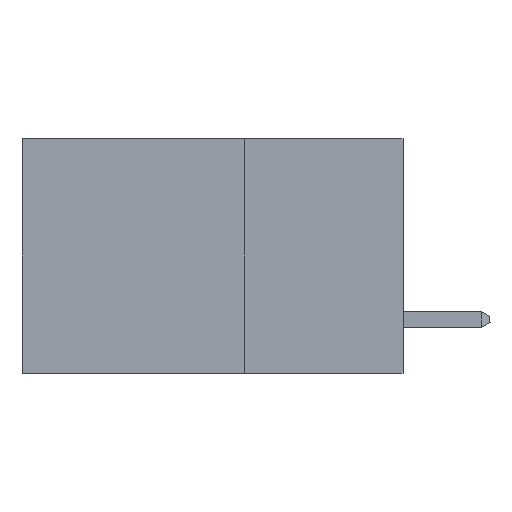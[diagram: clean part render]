
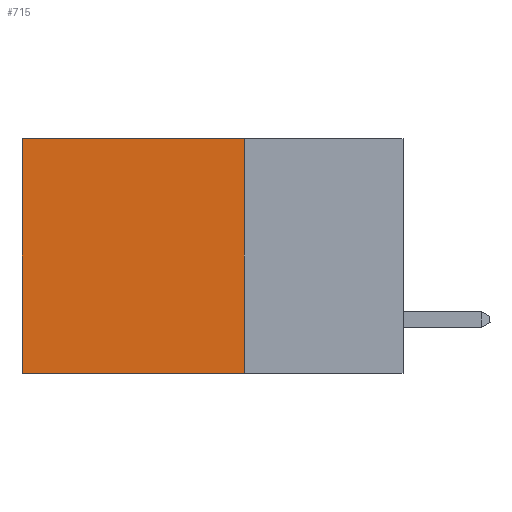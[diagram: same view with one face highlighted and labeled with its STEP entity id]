
A CAD part, left-side view. The second image highlights one B-rep face of the part: STEP entity #715.
In plain terms, the highlighted planar face has unit normal (-1, 0, 0).
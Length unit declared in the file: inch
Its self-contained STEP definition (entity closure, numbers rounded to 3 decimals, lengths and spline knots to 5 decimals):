
#684 = AXIS2_PLACEMENT_3D ( 'NONE', #42474, #21141, #42786 ) ;
#715 = ADVANCED_FACE ( 'NONE', ( #16308 ), #6292, .F. ) ;
#1144 = ORIENTED_EDGE ( 'NONE', *, *, #30104, .F. ) ;
#2700 = ORIENTED_EDGE ( 'NONE', *, *, #9098, .T. ) ;
#3795 = CARTESIAN_POINT ( 'NONE',  ( 0.2875, 0.25, 0. ) ) ;
#5429 = EDGE_CURVE ( 'NONE', #36516, #42840, #5952, .T. ) ;
#5790 = VERTEX_POINT ( 'NONE', #8399 ) ;
#5952 = LINE ( 'NONE', #10090, #33958 ) ;
#6292 = PLANE ( 'NONE',  #684 ) ;
#6444 = VECTOR ( 'NONE', #27448, 39.37008 ) ;
#6794 = CARTESIAN_POINT ( 'NONE',  ( 0.2875, 0.25, -0.37 ) ) ;
#8382 = CARTESIAN_POINT ( 'NONE',  ( 0.2875, 0.25, 0. ) ) ;
#8399 = CARTESIAN_POINT ( 'NONE',  ( 0.2875, 0.6, 0. ) ) ;
#9098 = EDGE_CURVE ( 'NONE', #36516, #5790, #30743, .T. ) ;
#10090 = CARTESIAN_POINT ( 'NONE',  ( 0.2875, 0.25, 0. ) ) ;
#16308 = FACE_OUTER_BOUND ( 'NONE', #29514, .T. ) ;
#16380 = CARTESIAN_POINT ( 'NONE',  ( 0.2875, 0.25, -0.37 ) ) ;
#17772 = ORIENTED_EDGE ( 'NONE', *, *, #23701, .T. ) ;
#19584 = CARTESIAN_POINT ( 'NONE',  ( 0.2875, 0.6, -0.37 ) ) ;
#21088 = CARTESIAN_POINT ( 'NONE',  ( 0.2875, 0.6, 0. ) ) ;
#21141 = DIRECTION ( 'NONE',  ( 1., 0., 0. ) ) ;
#21307 = VECTOR ( 'NONE', #22705, 39.37008 ) ;
#22705 = DIRECTION ( 'NONE',  ( 0., 1., 0. ) ) ;
#23375 = VERTEX_POINT ( 'NONE', #19584 ) ;
#23701 = EDGE_CURVE ( 'NONE', #5790, #23375, #35335, .T. ) ;
#27265 = DIRECTION ( 'NONE',  ( 0., 0., -1. ) ) ;
#27448 = DIRECTION ( 'NONE',  ( 0., 1., 0. ) ) ;
#28125 = DIRECTION ( 'NONE',  ( 0., 0., -1. ) ) ;
#29514 = EDGE_LOOP ( 'NONE', ( #17772, #1144, #42038, #2700 ) ) ;
#30104 = EDGE_CURVE ( 'NONE', #42840, #23375, #44038, .T. ) ;
#30743 = LINE ( 'NONE', #8382, #21307 ) ;
#33958 = VECTOR ( 'NONE', #27265, 39.37008 ) ;
#35335 = LINE ( 'NONE', #21088, #39256 ) ;
#36516 = VERTEX_POINT ( 'NONE', #3795 ) ;
#39256 = VECTOR ( 'NONE', #28125, 39.37008 ) ;
#42038 = ORIENTED_EDGE ( 'NONE', *, *, #5429, .F. ) ;
#42474 = CARTESIAN_POINT ( 'NONE',  ( 0.2875, 0.25, 0. ) ) ;
#42786 = DIRECTION ( 'NONE',  ( 0., 0., -1. ) ) ;
#42840 = VERTEX_POINT ( 'NONE', #6794 ) ;
#44038 = LINE ( 'NONE', #16380, #6444 ) ;
